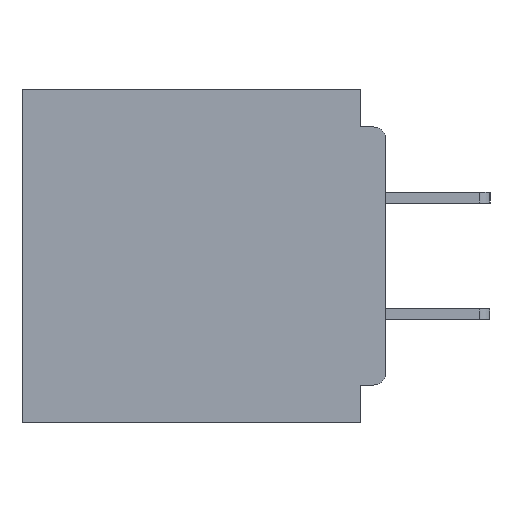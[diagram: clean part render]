
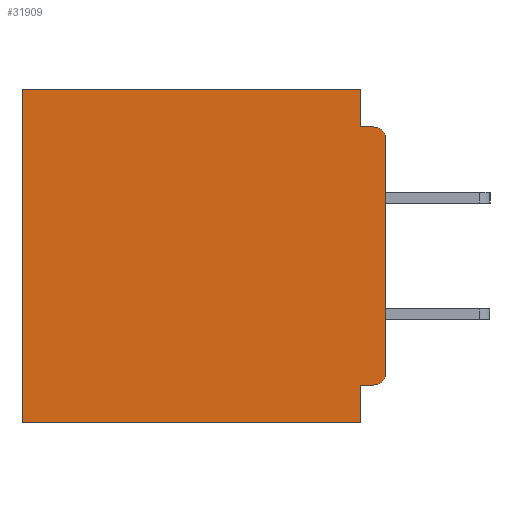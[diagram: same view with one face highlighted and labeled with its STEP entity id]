
A CAD part, left-side view. The second image highlights one B-rep face of the part: STEP entity #31909.
In plain terms, the highlighted planar face has unit normal (-1, 0, 0).
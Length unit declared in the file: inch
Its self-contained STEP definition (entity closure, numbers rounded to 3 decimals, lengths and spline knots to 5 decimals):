
#538 = VERTEX_POINT ( 'NONE', #29170 ) ;
#658 = CARTESIAN_POINT ( 'NONE',  ( 0.3, 0., -0.045 ) ) ;
#906 = ORIENTED_EDGE ( 'NONE', *, *, #34811, .F. ) ;
#949 = CIRCLE ( 'NONE', #30923, 0.015 ) ;
#1211 = VECTOR ( 'NONE', #28160, 39.37008 ) ;
#1322 = DIRECTION ( 'NONE',  ( 0., 0., -1. ) ) ;
#2268 = LINE ( 'NONE', #6197, #16258 ) ;
#2367 = LINE ( 'NONE', #5532, #32474 ) ;
#2796 = VECTOR ( 'NONE', #14631, 39.37008 ) ;
#3008 = EDGE_CURVE ( 'NONE', #21024, #4052, #949, .T. ) ;
#3477 = DIRECTION ( 'NONE',  ( 0., -1., 0. ) ) ;
#4052 = VERTEX_POINT ( 'NONE', #31147 ) ;
#4929 = LINE ( 'NONE', #22575, #34071 ) ;
#5129 = ORIENTED_EDGE ( 'NONE', *, *, #24387, .F. ) ;
#5364 = VERTEX_POINT ( 'NONE', #10081 ) ;
#5532 = CARTESIAN_POINT ( 'NONE',  ( 0.3, 0.031, 0. ) ) ;
#5834 = DIRECTION ( 'NONE',  ( 0., 0., -1. ) ) ;
#5935 = CARTESIAN_POINT ( 'NONE',  ( 0.3, 0.015, -0.06 ) ) ;
#6076 = VECTOR ( 'NONE', #3477, 39.37008 ) ;
#6197 = CARTESIAN_POINT ( 'NONE',  ( 0.3, 0., 0. ) ) ;
#6364 = CARTESIAN_POINT ( 'NONE',  ( 0.3, 0.015, -0.355 ) ) ;
#6856 = VECTOR ( 'NONE', #9437, 39.37008 ) ;
#6899 = ORIENTED_EDGE ( 'NONE', *, *, #13397, .F. ) ;
#7712 = LINE ( 'NONE', #23441, #6856 ) ;
#8587 = CARTESIAN_POINT ( 'NONE',  ( 0.3, 0., -0.355 ) ) ;
#8729 = DIRECTION ( 'NONE',  ( 0., 0., -1. ) ) ;
#8959 = CARTESIAN_POINT ( 'NONE',  ( 0.3, 0.031, 0. ) ) ;
#9042 = DIRECTION ( 'NONE',  ( 0., 0., -1. ) ) ;
#9395 = LINE ( 'NONE', #31743, #2796 ) ;
#9437 = DIRECTION ( 'NONE',  ( 0., 1., 0. ) ) ;
#10081 = CARTESIAN_POINT ( 'NONE',  ( 0.3, 0.031, -0.045 ) ) ;
#10713 = DIRECTION ( 'NONE',  ( -1., 0., 0. ) ) ;
#11456 = CARTESIAN_POINT ( 'NONE',  ( 0.3, 0., -0.4 ) ) ;
#11482 = EDGE_CURVE ( 'NONE', #21024, #538, #14329, .T. ) ;
#11611 = CARTESIAN_POINT ( 'NONE',  ( 0.3, 0., -0.06 ) ) ;
#12601 = AXIS2_PLACEMENT_3D ( 'NONE', #5935, #25613, #8729 ) ;
#13159 = ORIENTED_EDGE ( 'NONE', *, *, #23059, .F. ) ;
#13397 = EDGE_CURVE ( 'NONE', #29534, #30008, #7712, .T. ) ;
#14229 = PLANE ( 'NONE',  #23550 ) ;
#14329 = LINE ( 'NONE', #8587, #1211 ) ;
#14476 = ORIENTED_EDGE ( 'NONE', *, *, #3008, .T. ) ;
#14494 = CARTESIAN_POINT ( 'NONE',  ( 0.3, 0., -0.4 ) ) ;
#14631 = DIRECTION ( 'NONE',  ( 0., 0., -1. ) ) ;
#15496 = VERTEX_POINT ( 'NONE', #8959 ) ;
#16258 = VECTOR ( 'NONE', #28805, 39.37008 ) ;
#16521 = EDGE_CURVE ( 'NONE', #538, #29534, #9395, .T. ) ;
#17074 = DIRECTION ( 'NONE',  ( 0., 0., -1. ) ) ;
#20168 = CIRCLE ( 'NONE', #12601, 0.015 ) ;
#21024 = VERTEX_POINT ( 'NONE', #6364 ) ;
#21145 = VERTEX_POINT ( 'NONE', #26700 ) ;
#22575 = CARTESIAN_POINT ( 'NONE',  ( 0.3, 0.437, -0.4 ) ) ;
#23036 = ORIENTED_EDGE ( 'NONE', *, *, #11482, .F. ) ;
#23059 = EDGE_CURVE ( 'NONE', #5364, #21145, #28611, .T. ) ;
#23312 = ORIENTED_EDGE ( 'NONE', *, *, #36036, .T. ) ;
#23441 = CARTESIAN_POINT ( 'NONE',  ( 0.3, 0., -0.4 ) ) ;
#23550 = AXIS2_PLACEMENT_3D ( 'NONE', #11456, #34110, #17074 ) ;
#23922 = CARTESIAN_POINT ( 'NONE',  ( 0.3, 0.437, 0. ) ) ;
#24387 = EDGE_CURVE ( 'NONE', #31293, #4052, #28115, .T. ) ;
#25188 = DIRECTION ( 'NONE',  ( 0., 0., -1. ) ) ;
#25613 = DIRECTION ( 'NONE',  ( -1., 0., 0. ) ) ;
#26700 = CARTESIAN_POINT ( 'NONE',  ( 0.3, 0.015, -0.045 ) ) ;
#27221 = EDGE_LOOP ( 'NONE', ( #5129, #35135, #13159, #906, #36004, #23312, #6899, #33602, #23036, #14476 ) ) ;
#27222 = FACE_OUTER_BOUND ( 'NONE', #27221, .T. ) ;
#27528 = EDGE_CURVE ( 'NONE', #31293, #21145, #20168, .T. ) ;
#27779 = CARTESIAN_POINT ( 'NONE',  ( 0.3, 0.437, -0.4 ) ) ;
#28115 = LINE ( 'NONE', #14494, #34698 ) ;
#28160 = DIRECTION ( 'NONE',  ( 0., 1., 0. ) ) ;
#28611 = LINE ( 'NONE', #658, #6076 ) ;
#28805 = DIRECTION ( 'NONE',  ( 0., 1., 0. ) ) ;
#29170 = CARTESIAN_POINT ( 'NONE',  ( 0.3, 0.031, -0.355 ) ) ;
#29534 = VERTEX_POINT ( 'NONE', #31187 ) ;
#30008 = VERTEX_POINT ( 'NONE', #27779 ) ;
#30923 = AXIS2_PLACEMENT_3D ( 'NONE', #32695, #10713, #1322 ) ;
#31147 = CARTESIAN_POINT ( 'NONE',  ( 0.3, 0., -0.34 ) ) ;
#31187 = CARTESIAN_POINT ( 'NONE',  ( 0.3, 0.031, -0.4 ) ) ;
#31293 = VERTEX_POINT ( 'NONE', #11611 ) ;
#31520 = VERTEX_POINT ( 'NONE', #23922 ) ;
#31743 = CARTESIAN_POINT ( 'NONE',  ( 0.3, 0.031, -0.4 ) ) ;
#31909 = ADVANCED_FACE ( 'NONE', ( #27222 ), #14229, .F. ) ;
#32474 = VECTOR ( 'NONE', #25188, 39.37008 ) ;
#32695 = CARTESIAN_POINT ( 'NONE',  ( 0.3, 0.015, -0.34 ) ) ;
#33602 = ORIENTED_EDGE ( 'NONE', *, *, #16521, .F. ) ;
#34071 = VECTOR ( 'NONE', #5834, 39.37008 ) ;
#34110 = DIRECTION ( 'NONE',  ( 1., 0., 0. ) ) ;
#34698 = VECTOR ( 'NONE', #9042, 39.37008 ) ;
#34811 = EDGE_CURVE ( 'NONE', #15496, #5364, #2367, .T. ) ;
#35135 = ORIENTED_EDGE ( 'NONE', *, *, #27528, .T. ) ;
#36004 = ORIENTED_EDGE ( 'NONE', *, *, #36138, .T. ) ;
#36036 = EDGE_CURVE ( 'NONE', #31520, #30008, #4929, .T. ) ;
#36138 = EDGE_CURVE ( 'NONE', #15496, #31520, #2268, .T. ) ;
